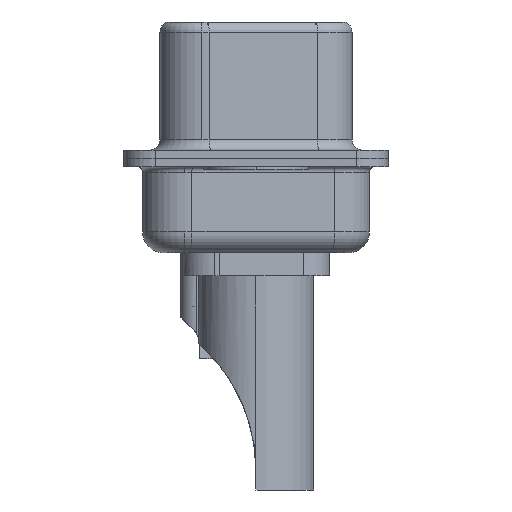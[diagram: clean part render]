
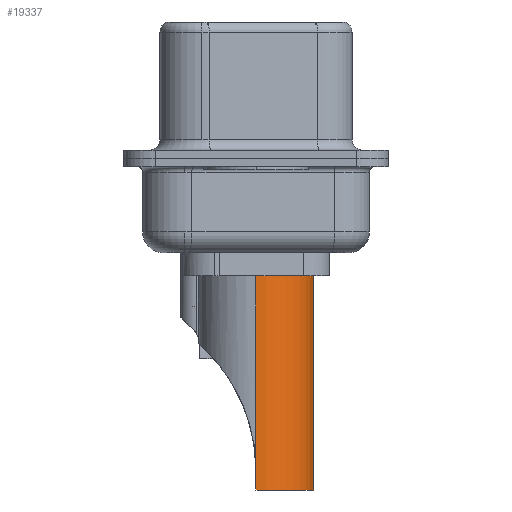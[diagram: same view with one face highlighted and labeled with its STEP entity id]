
A CAD part, left-side view. The second image highlights one B-rep face of the part: STEP entity #19337.
In plain terms, the highlighted cylindrical face has radius 2.75 mm (diameter 5.5 mm), a partial arc.
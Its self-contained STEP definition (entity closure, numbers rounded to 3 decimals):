
#433 = DIRECTION ( 'NONE',  ( 1., 0., 0. ) ) ;
#697 = AXIS2_PLACEMENT_3D ( 'NONE', #20757, #11169, #1368 ) ;
#1368 = DIRECTION ( 'NONE',  ( 1., 0., 0. ) ) ;
#1979 = ORIENTED_EDGE ( 'NONE', *, *, #2143, .T. ) ;
#2143 = EDGE_CURVE ( 'NONE', #12472, #9712, #6603, .T. ) ;
#3179 = CARTESIAN_POINT ( 'NONE',  ( -2.75, 0., -8.7 ) ) ;
#3416 = DIRECTION ( 'NONE',  ( 0., 0., 1. ) ) ;
#3633 = CARTESIAN_POINT ( 'NONE',  ( 2.75, 0., 4.234 ) ) ;
#3901 = AXIS2_PLACEMENT_3D ( 'NONE', #19867, #10329, #433 ) ;
#3914 = DIRECTION ( 'NONE',  ( 0., 0., 1. ) ) ;
#4278 = VERTEX_POINT ( 'NONE', #18199 ) ;
#4716 = VECTOR ( 'NONE', #3416, 1000. ) ;
#4822 = VECTOR ( 'NONE', #14939, 1000. ) ;
#5702 = ORIENTED_EDGE ( 'NONE', *, *, #15883, .F. ) ;
#5798 = ORIENTED_EDGE ( 'NONE', *, *, #11184, .F. ) ;
#6113 = VECTOR ( 'NONE', #7414, 1000. ) ;
#6177 = CYLINDRICAL_SURFACE ( 'NONE', #9220, 2.75 ) ;
#6603 = LINE ( 'NONE', #9384, #6113 ) ;
#6618 = VERTEX_POINT ( 'NONE', #6968 ) ;
#6968 = CARTESIAN_POINT ( 'NONE',  ( 2.75, 0., -7.764 ) ) ;
#7414 = DIRECTION ( 'NONE',  ( 0., 0., -1. ) ) ;
#7994 = VERTEX_POINT ( 'NONE', #16969 ) ;
#8238 = CARTESIAN_POINT ( 'NONE',  ( -2.75, 0., 4.234 ) ) ;
#8408 = CIRCLE ( 'NONE', #697, 2.75 ) ;
#9149 = LINE ( 'NONE', #3633, #4822 ) ;
#9220 = AXIS2_PLACEMENT_3D ( 'NONE', #15203, #3914, #19921 ) ;
#9316 = DIRECTION ( 'NONE',  ( 0., 0., -1. ) ) ;
#9384 = CARTESIAN_POINT ( 'NONE',  ( -2.75, 0., -8.7 ) ) ;
#9712 = VERTEX_POINT ( 'NONE', #3179 ) ;
#10306 = VERTEX_POINT ( 'NONE', #14686 ) ;
#10329 = DIRECTION ( 'NONE',  ( 0., 0., 1. ) ) ;
#10339 = EDGE_LOOP ( 'NONE', ( #16174, #1979, #16446, #5702, #11966, #5798 ) ) ;
#11169 = DIRECTION ( 'NONE',  ( 0., 0., 1. ) ) ;
#11184 = EDGE_CURVE ( 'NONE', #10306, #7994, #8408, .T. ) ;
#11302 = EDGE_CURVE ( 'NONE', #6618, #7994, #9149, .T. ) ;
#11966 = ORIENTED_EDGE ( 'NONE', *, *, #11302, .T. ) ;
#12472 = VERTEX_POINT ( 'NONE', #19339 ) ;
#12933 = CIRCLE ( 'NONE', #3901, 2.75 ) ;
#14259 = VECTOR ( 'NONE', #9316, 1000. ) ;
#14686 = CARTESIAN_POINT ( 'NONE',  ( -2.75, 0., 1.5 ) ) ;
#14917 = EDGE_CURVE ( 'NONE', #12472, #10306, #17540, .T. ) ;
#14939 = DIRECTION ( 'NONE',  ( 0., 0., 1. ) ) ;
#15203 = CARTESIAN_POINT ( 'NONE',  ( 0., 0., 4.234 ) ) ;
#15246 = LINE ( 'NONE', #18872, #14259 ) ;
#15883 = EDGE_CURVE ( 'NONE', #6618, #4278, #15246, .T. ) ;
#16174 = ORIENTED_EDGE ( 'NONE', *, *, #14917, .F. ) ;
#16446 = ORIENTED_EDGE ( 'NONE', *, *, #20555, .T. ) ;
#16969 = CARTESIAN_POINT ( 'NONE',  ( 2.75, 0., 1.5 ) ) ;
#17540 = LINE ( 'NONE', #8238, #4716 ) ;
#18199 = CARTESIAN_POINT ( 'NONE',  ( 2.75, 0., -8.7 ) ) ;
#18872 = CARTESIAN_POINT ( 'NONE',  ( 2.75, 0., -8.7 ) ) ;
#18955 = FACE_OUTER_BOUND ( 'NONE', #10339, .T. ) ;
#19337 = ADVANCED_FACE ( 'NONE', ( #18955 ), #6177, .T. ) ;
#19339 = CARTESIAN_POINT ( 'NONE',  ( -2.75, 0., -7.764 ) ) ;
#19867 = CARTESIAN_POINT ( 'NONE',  ( 0., 0., -8.7 ) ) ;
#19921 = DIRECTION ( 'NONE',  ( 1., 0., 0. ) ) ;
#20555 = EDGE_CURVE ( 'NONE', #9712, #4278, #12933, .T. ) ;
#20757 = CARTESIAN_POINT ( 'NONE',  ( 0., 0., 1.5 ) ) ;
